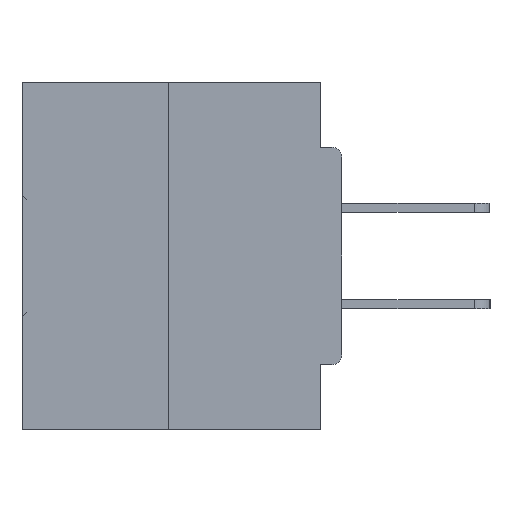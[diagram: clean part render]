
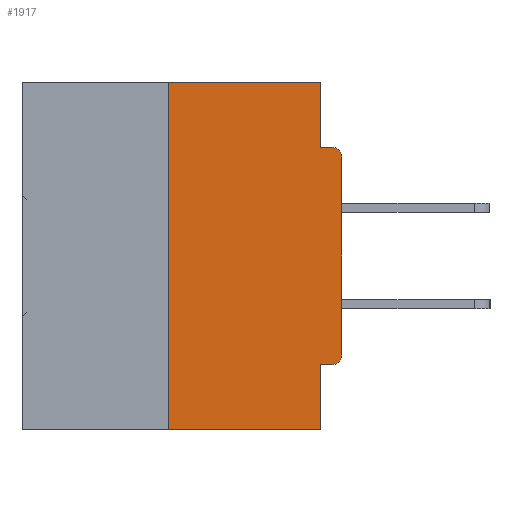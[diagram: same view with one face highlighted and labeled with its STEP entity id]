
A CAD part, left-side view. The second image highlights one B-rep face of the part: STEP entity #1917.
In plain terms, the highlighted planar face has unit normal (-1, 0, 0).
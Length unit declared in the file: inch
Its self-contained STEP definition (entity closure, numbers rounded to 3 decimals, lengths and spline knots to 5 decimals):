
#539 = DIRECTION ( 'NONE',  ( -1., 0., 0. ) ) ;
#909 = CARTESIAN_POINT ( 'NONE',  ( 0., 0.031, -0.0935 ) ) ;
#983 = CARTESIAN_POINT ( 'NONE',  ( 0., 0., -0.3915 ) ) ;
#1917 = ADVANCED_FACE ( 'NONE', ( #34552 ), #3446, .F. ) ;
#2062 = CARTESIAN_POINT ( 'NONE',  ( 0., 0.031, -0.4065 ) ) ;
#2331 = EDGE_CURVE ( 'NONE', #26156, #23283, #37225, .T. ) ;
#3075 = VERTEX_POINT ( 'NONE', #9158 ) ;
#3163 = DIRECTION ( 'NONE',  ( 0., 0., 1. ) ) ;
#3446 = PLANE ( 'NONE',  #21356 ) ;
#3889 = LINE ( 'NONE', #6864, #24196 ) ;
#4641 = VECTOR ( 'NONE', #35842, 39.37008 ) ;
#4812 = VERTEX_POINT ( 'NONE', #26356 ) ;
#5587 = ORIENTED_EDGE ( 'NONE', *, *, #33238, .T. ) ;
#6088 = CARTESIAN_POINT ( 'NONE',  ( 0., 0.46, 0. ) ) ;
#6864 = CARTESIAN_POINT ( 'NONE',  ( 0., 0.031, -0.5 ) ) ;
#7016 = DIRECTION ( 'NONE',  ( 0., 0., -1. ) ) ;
#8010 = VERTEX_POINT ( 'NONE', #983 ) ;
#8014 = EDGE_CURVE ( 'NONE', #4812, #8010, #21156, .T. ) ;
#8992 = CIRCLE ( 'NONE', #24331, 0.015 ) ;
#9158 = CARTESIAN_POINT ( 'NONE',  ( 0., 0.25, 0. ) ) ;
#9188 = DIRECTION ( 'NONE',  ( 0., 0., -1. ) ) ;
#9308 = CARTESIAN_POINT ( 'NONE',  ( 0., 0., -0.0935 ) ) ;
#9366 = EDGE_LOOP ( 'NONE', ( #38042, #28482, #10102, #35895, #23954, #35741, #5587, #37061, #13525, #33928 ) ) ;
#9984 = EDGE_CURVE ( 'NONE', #16421, #12390, #39517, .T. ) ;
#10102 = ORIENTED_EDGE ( 'NONE', *, *, #9984, .T. ) ;
#12083 = EDGE_CURVE ( 'NONE', #3075, #21536, #27604, .T. ) ;
#12309 = CARTESIAN_POINT ( 'NONE',  ( 0., 0.25, 0. ) ) ;
#12390 = VERTEX_POINT ( 'NONE', #25789 ) ;
#12776 = DIRECTION ( 'NONE',  ( 1., 0., 0. ) ) ;
#13525 = ORIENTED_EDGE ( 'NONE', *, *, #2331, .F. ) ;
#13912 = CARTESIAN_POINT ( 'NONE',  ( 0., 0.015, -0.3915 ) ) ;
#16421 = VERTEX_POINT ( 'NONE', #28426 ) ;
#17288 = DIRECTION ( 'NONE',  ( 0., 0., -1. ) ) ;
#17289 = CARTESIAN_POINT ( 'NONE',  ( 0., 0.46, 0. ) ) ;
#19347 = DIRECTION ( 'NONE',  ( 0., -1., 0. ) ) ;
#19762 = VECTOR ( 'NONE', #26952, 39.37008 ) ;
#20685 = EDGE_CURVE ( 'NONE', #38551, #23283, #8992, .T. ) ;
#21156 = CIRCLE ( 'NONE', #26984, 0.015 ) ;
#21356 = AXIS2_PLACEMENT_3D ( 'NONE', #17289, #12776, #26632 ) ;
#21466 = EDGE_CURVE ( 'NONE', #4812, #32039, #35602, .T. ) ;
#21536 = VERTEX_POINT ( 'NONE', #39462 ) ;
#22242 = VECTOR ( 'NONE', #32771, 39.37008 ) ;
#22995 = LINE ( 'NONE', #40219, #22242 ) ;
#23283 = VERTEX_POINT ( 'NONE', #31361 ) ;
#23722 = EDGE_CURVE ( 'NONE', #21536, #26156, #30876, .T. ) ;
#23954 = ORIENTED_EDGE ( 'NONE', *, *, #21466, .F. ) ;
#24196 = VECTOR ( 'NONE', #17288, 39.37008 ) ;
#24331 = AXIS2_PLACEMENT_3D ( 'NONE', #25775, #40252, #9188 ) ;
#24368 = VECTOR ( 'NONE', #7016, 39.37008 ) ;
#25295 = CARTESIAN_POINT ( 'NONE',  ( 0., 0., -0.1085 ) ) ;
#25485 = CARTESIAN_POINT ( 'NONE',  ( 0., 0.46, -0.5 ) ) ;
#25775 = CARTESIAN_POINT ( 'NONE',  ( 0., 0.015, -0.1085 ) ) ;
#25789 = CARTESIAN_POINT ( 'NONE',  ( 0., 0.031, -0.5 ) ) ;
#26156 = VERTEX_POINT ( 'NONE', #909 ) ;
#26215 = VECTOR ( 'NONE', #3163, 39.37008 ) ;
#26356 = CARTESIAN_POINT ( 'NONE',  ( 0., 0.015, -0.4065 ) ) ;
#26632 = DIRECTION ( 'NONE',  ( 0., 0., -1. ) ) ;
#26952 = DIRECTION ( 'NONE',  ( 0., -1., 0. ) ) ;
#26984 = AXIS2_PLACEMENT_3D ( 'NONE', #13912, #539, #28648 ) ;
#27604 = LINE ( 'NONE', #6088, #19762 ) ;
#28426 = CARTESIAN_POINT ( 'NONE',  ( 0., 0.25, -0.5 ) ) ;
#28482 = ORIENTED_EDGE ( 'NONE', *, *, #35600, .F. ) ;
#28648 = DIRECTION ( 'NONE',  ( 0., 0., -1. ) ) ;
#29279 = CARTESIAN_POINT ( 'NONE',  ( 0., 0., -0.4065 ) ) ;
#30085 = EDGE_CURVE ( 'NONE', #32039, #12390, #3889, .T. ) ;
#30876 = LINE ( 'NONE', #44695, #24368 ) ;
#31361 = CARTESIAN_POINT ( 'NONE',  ( 0., 0.015, -0.0935 ) ) ;
#32039 = VERTEX_POINT ( 'NONE', #2062 ) ;
#32771 = DIRECTION ( 'NONE',  ( 0., 0., 1. ) ) ;
#33238 = EDGE_CURVE ( 'NONE', #8010, #38551, #22995, .T. ) ;
#33928 = ORIENTED_EDGE ( 'NONE', *, *, #23722, .F. ) ;
#34552 = FACE_OUTER_BOUND ( 'NONE', #9366, .T. ) ;
#35600 = EDGE_CURVE ( 'NONE', #16421, #3075, #44467, .T. ) ;
#35602 = LINE ( 'NONE', #29279, #4641 ) ;
#35741 = ORIENTED_EDGE ( 'NONE', *, *, #8014, .T. ) ;
#35842 = DIRECTION ( 'NONE',  ( 0., 1., 0. ) ) ;
#35895 = ORIENTED_EDGE ( 'NONE', *, *, #30085, .F. ) ;
#37050 = VECTOR ( 'NONE', #19347, 39.37008 ) ;
#37061 = ORIENTED_EDGE ( 'NONE', *, *, #20685, .T. ) ;
#37225 = LINE ( 'NONE', #9308, #42381 ) ;
#38042 = ORIENTED_EDGE ( 'NONE', *, *, #12083, .F. ) ;
#38551 = VERTEX_POINT ( 'NONE', #25295 ) ;
#39462 = CARTESIAN_POINT ( 'NONE',  ( 0., 0.031, 0. ) ) ;
#39517 = LINE ( 'NONE', #25485, #37050 ) ;
#40219 = CARTESIAN_POINT ( 'NONE',  ( 0., 0., 0. ) ) ;
#40252 = DIRECTION ( 'NONE',  ( -1., 0., 0. ) ) ;
#40381 = DIRECTION ( 'NONE',  ( 0., -1., 0. ) ) ;
#42381 = VECTOR ( 'NONE', #40381, 39.37008 ) ;
#44467 = LINE ( 'NONE', #12309, #26215 ) ;
#44695 = CARTESIAN_POINT ( 'NONE',  ( 0., 0.031, 0. ) ) ;
